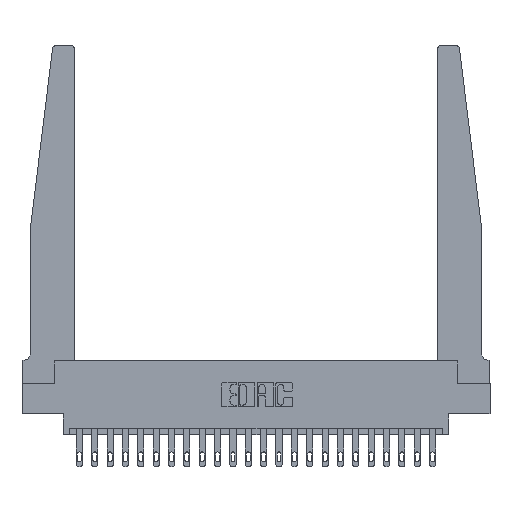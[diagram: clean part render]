
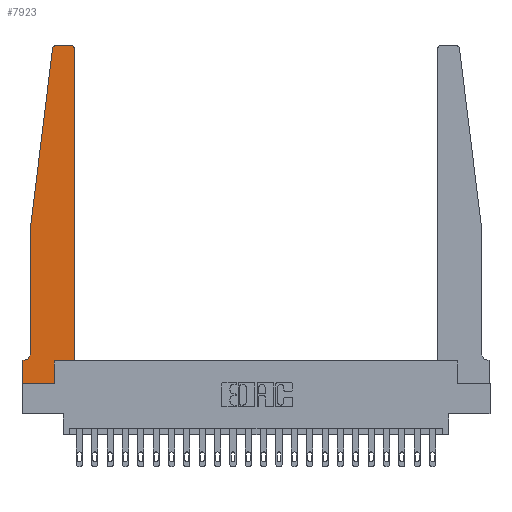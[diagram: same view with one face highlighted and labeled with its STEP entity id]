
A CAD part, top view. The second image highlights one B-rep face of the part: STEP entity #7923.
In plain terms, the highlighted planar face has unit normal (0, 0, 1).
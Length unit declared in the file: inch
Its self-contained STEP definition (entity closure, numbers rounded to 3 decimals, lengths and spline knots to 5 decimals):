
#141 = CARTESIAN_POINT ( 'NONE',  ( 0.395, 2.75, 0.37 ) ) ;
#358 = FACE_OUTER_BOUND ( 'NONE', #7919, .T. ) ;
#973 = CARTESIAN_POINT ( 'NONE',  ( 0.065, 1.25, 0.37 ) ) ;
#1357 = VECTOR ( 'NONE', #2628, 39.37008 ) ;
#1392 = CARTESIAN_POINT ( 'NONE',  ( 0.27653, 2.75, 0.37 ) ) ;
#1424 = ORIENTED_EDGE ( 'NONE', *, *, #4599, .T. ) ;
#1455 = VECTOR ( 'NONE', #5330, 39.37008 ) ;
#1613 = VECTOR ( 'NONE', #17219, 39.37008 ) ;
#1880 = CARTESIAN_POINT ( 'NONE',  ( 0.2605, 0.18, 0.37 ) ) ;
#1970 = DIRECTION ( 'NONE',  ( 0., 1., 0. ) ) ;
#2109 = VECTOR ( 'NONE', #18913, 39.37008 ) ;
#2241 = ORIENTED_EDGE ( 'NONE', *, *, #22141, .T. ) ;
#2335 = VERTEX_POINT ( 'NONE', #1880 ) ;
#2628 = DIRECTION ( 'NONE',  ( 0., -1., 0. ) ) ;
#2741 = CARTESIAN_POINT ( 'NONE',  ( 0.2605, 0.18, 0.37 ) ) ;
#2821 = VERTEX_POINT ( 'NONE', #10923 ) ;
#2930 = VERTEX_POINT ( 'NONE', #4090 ) ;
#4090 = CARTESIAN_POINT ( 'NONE',  ( 0., 0., 0.37 ) ) ;
#4125 = VERTEX_POINT ( 'NONE', #1392 ) ;
#4126 = PLANE ( 'NONE',  #20630 ) ;
#4570 = DIRECTION ( 'NONE',  ( -1., 0., 0. ) ) ;
#4599 = EDGE_CURVE ( 'NONE', #22368, #16066, #11754, .T. ) ;
#4694 = CARTESIAN_POINT ( 'NONE',  ( 0.25, 2.75, 0.37 ) ) ;
#4799 = CARTESIAN_POINT ( 'NONE',  ( 0., 0.1875, 0.37 ) ) ;
#5292 = LINE ( 'NONE', #9047, #9226 ) ;
#5330 = DIRECTION ( 'NONE',  ( 1., 0., 0. ) ) ;
#5466 = ORIENTED_EDGE ( 'NONE', *, *, #6440, .T. ) ;
#6440 = EDGE_CURVE ( 'NONE', #7897, #6858, #5292, .T. ) ;
#6508 = DIRECTION ( 'NONE',  ( 0., -1., 0. ) ) ;
#6858 = VERTEX_POINT ( 'NONE', #19800 ) ;
#6919 = CARTESIAN_POINT ( 'NONE',  ( 0.24675, 2.72367, 0.37 ) ) ;
#7478 = DIRECTION ( 'NONE',  ( 0., 0., 1. ) ) ;
#7547 = DIRECTION ( 'NONE',  ( 0., 0., 1. ) ) ;
#7608 = EDGE_CURVE ( 'NONE', #11733, #2930, #9918, .T. ) ;
#7643 = DIRECTION ( 'NONE',  ( -0.122, -0.992, 0. ) ) ;
#7823 = AXIS2_PLACEMENT_3D ( 'NONE', #21820, #18376, #11136 ) ;
#7897 = VERTEX_POINT ( 'NONE', #21522 ) ;
#7919 = EDGE_LOOP ( 'NONE', ( #2241, #8579, #1424, #15055, #20982, #18444, #11231, #21995, #9995, #17522, #5466, #17760 ) ) ;
#7923 = ADVANCED_FACE ( 'NONE', ( #358 ), #4126, .T. ) ;
#8387 = CARTESIAN_POINT ( 'NONE',  ( 0., 0., 0.37 ) ) ;
#8568 = VECTOR ( 'NONE', #6508, 39.37008 ) ;
#8579 = ORIENTED_EDGE ( 'NONE', *, *, #16372, .T. ) ;
#8612 = CIRCLE ( 'NONE', #10117, 0.03 ) ;
#8696 = LINE ( 'NONE', #11760, #1613 ) ;
#8982 = LINE ( 'NONE', #21764, #1455 ) ;
#9047 = CARTESIAN_POINT ( 'NONE',  ( 0.425, 0.18, 0.37 ) ) ;
#9079 = DIRECTION ( 'NONE',  ( 1., 0., 0. ) ) ;
#9226 = VECTOR ( 'NONE', #1970, 39.37008 ) ;
#9412 = VERTEX_POINT ( 'NONE', #141 ) ;
#9918 = LINE ( 'NONE', #8387, #1357 ) ;
#9922 = VERTEX_POINT ( 'NONE', #21511 ) ;
#9995 = ORIENTED_EDGE ( 'NONE', *, *, #16916, .T. ) ;
#10017 = AXIS2_PLACEMENT_3D ( 'NONE', #18235, #7478, #22033 ) ;
#10080 = CARTESIAN_POINT ( 'NONE',  ( 0.065, 0.1875, 0.37 ) ) ;
#10117 = AXIS2_PLACEMENT_3D ( 'NONE', #17494, #23190, #13945 ) ;
#10157 = EDGE_CURVE ( 'NONE', #2930, #22361, #8696, .T. ) ;
#10923 = CARTESIAN_POINT ( 'NONE',  ( 0.015, 0.1875, 0.37 ) ) ;
#11136 = DIRECTION ( 'NONE',  ( -1., 0., 0. ) ) ;
#11231 = ORIENTED_EDGE ( 'NONE', *, *, #7608, .T. ) ;
#11575 = CIRCLE ( 'NONE', #10017, 0.03 ) ;
#11733 = VERTEX_POINT ( 'NONE', #4799 ) ;
#11754 = LINE ( 'NONE', #13197, #18855 ) ;
#11760 = CARTESIAN_POINT ( 'NONE',  ( 0., 0., 0.37 ) ) ;
#12163 = LINE ( 'NONE', #973, #8568 ) ;
#13197 = CARTESIAN_POINT ( 'NONE',  ( 0.065, 1.25, 0.37 ) ) ;
#13399 = LINE ( 'NONE', #10080, #19073 ) ;
#13945 = DIRECTION ( 'NONE',  ( 1., 0., 0. ) ) ;
#14743 = EDGE_CURVE ( 'NONE', #2821, #11733, #13399, .T. ) ;
#14876 = CARTESIAN_POINT ( 'NONE',  ( 0., 0.1875, 0.37 ) ) ;
#15055 = ORIENTED_EDGE ( 'NONE', *, *, #19862, .T. ) ;
#15543 = LINE ( 'NONE', #4694, #18454 ) ;
#16066 = VERTEX_POINT ( 'NONE', #20860 ) ;
#16372 = EDGE_CURVE ( 'NONE', #4125, #22368, #11575, .T. ) ;
#16916 = EDGE_CURVE ( 'NONE', #22361, #2335, #20584, .T. ) ;
#17179 = DIRECTION ( 'NONE',  ( -1., 0., 0. ) ) ;
#17219 = DIRECTION ( 'NONE',  ( 1., 0., 0. ) ) ;
#17494 = CARTESIAN_POINT ( 'NONE',  ( 0.395, 2.72, 0.37 ) ) ;
#17522 = ORIENTED_EDGE ( 'NONE', *, *, #21380, .T. ) ;
#17760 = ORIENTED_EDGE ( 'NONE', *, *, #21208, .T. ) ;
#18141 = CARTESIAN_POINT ( 'NONE',  ( 0.2605, 0., 0.37 ) ) ;
#18235 = CARTESIAN_POINT ( 'NONE',  ( 0.27653, 2.72, 0.37 ) ) ;
#18376 = DIRECTION ( 'NONE',  ( 0., 0., -1. ) ) ;
#18444 = ORIENTED_EDGE ( 'NONE', *, *, #14743, .T. ) ;
#18454 = VECTOR ( 'NONE', #4570, 39.37008 ) ;
#18855 = VECTOR ( 'NONE', #7643, 39.37008 ) ;
#18913 = DIRECTION ( 'NONE',  ( 0., 1., 0. ) ) ;
#19073 = VECTOR ( 'NONE', #17179, 39.37008 ) ;
#19800 = CARTESIAN_POINT ( 'NONE',  ( 0.425, 2.72, 0.37 ) ) ;
#19862 = EDGE_CURVE ( 'NONE', #16066, #9922, #12163, .T. ) ;
#20584 = LINE ( 'NONE', #2741, #2109 ) ;
#20594 = EDGE_CURVE ( 'NONE', #9922, #2821, #21441, .T. ) ;
#20630 = AXIS2_PLACEMENT_3D ( 'NONE', #14876, #7547, #9079 ) ;
#20860 = CARTESIAN_POINT ( 'NONE',  ( 0.065, 1.25, 0.37 ) ) ;
#20982 = ORIENTED_EDGE ( 'NONE', *, *, #20594, .T. ) ;
#21208 = EDGE_CURVE ( 'NONE', #6858, #9412, #8612, .T. ) ;
#21380 = EDGE_CURVE ( 'NONE', #2335, #7897, #8982, .T. ) ;
#21441 = CIRCLE ( 'NONE', #7823, 0.05 ) ;
#21511 = CARTESIAN_POINT ( 'NONE',  ( 0.065, 0.2375, 0.37 ) ) ;
#21522 = CARTESIAN_POINT ( 'NONE',  ( 0.425, 0.18, 0.37 ) ) ;
#21764 = CARTESIAN_POINT ( 'NONE',  ( 0.425, 0.18, 0.37 ) ) ;
#21820 = CARTESIAN_POINT ( 'NONE',  ( 0.015, 0.2375, 0.37 ) ) ;
#21995 = ORIENTED_EDGE ( 'NONE', *, *, #10157, .T. ) ;
#22033 = DIRECTION ( 'NONE',  ( 1., 0., 0. ) ) ;
#22141 = EDGE_CURVE ( 'NONE', #9412, #4125, #15543, .T. ) ;
#22361 = VERTEX_POINT ( 'NONE', #18141 ) ;
#22368 = VERTEX_POINT ( 'NONE', #6919 ) ;
#23190 = DIRECTION ( 'NONE',  ( 0., 0., 1. ) ) ;
